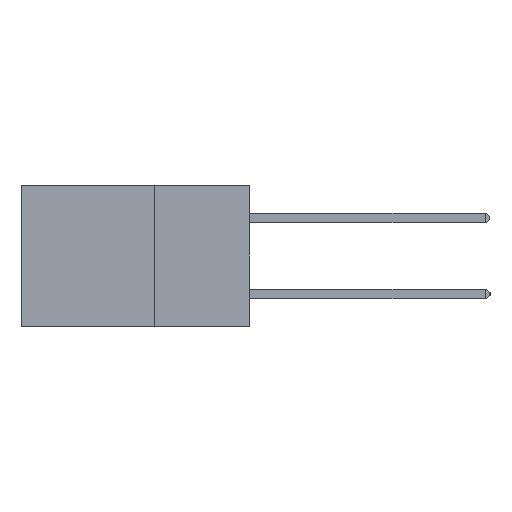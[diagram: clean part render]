
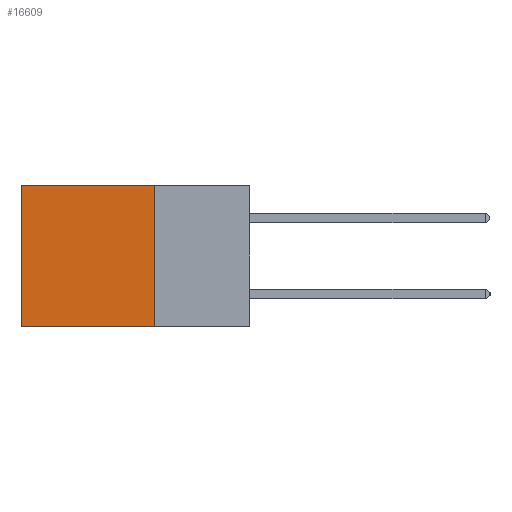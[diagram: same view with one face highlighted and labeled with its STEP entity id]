
A CAD part, left-side view. The second image highlights one B-rep face of the part: STEP entity #16609.
In plain terms, the highlighted planar face has unit normal (-1, 0, 0).
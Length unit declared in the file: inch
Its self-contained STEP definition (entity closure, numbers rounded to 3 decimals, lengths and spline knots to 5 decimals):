
#567 = VECTOR ( 'NONE', #21904, 39.37008 ) ;
#696 = ORIENTED_EDGE ( 'NONE', *, *, #16362, .F. ) ;
#1160 = ORIENTED_EDGE ( 'NONE', *, *, #2535, .T. ) ;
#2535 = EDGE_CURVE ( 'NONE', #18278, #21235, #11770, .T. ) ;
#5441 = FACE_OUTER_BOUND ( 'NONE', #7882, .T. ) ;
#5723 = VECTOR ( 'NONE', #8265, 39.37008 ) ;
#5736 = AXIS2_PLACEMENT_3D ( 'NONE', #21163, #8932, #21237 ) ;
#5966 = VECTOR ( 'NONE', #14530, 39.37008 ) ;
#7166 = PLANE ( 'NONE',  #5736 ) ;
#7882 = EDGE_LOOP ( 'NONE', ( #8597, #20189, #696, #1160 ) ) ;
#8265 = DIRECTION ( 'NONE',  ( 0., 0., -1. ) ) ;
#8451 = CARTESIAN_POINT ( 'NONE',  ( 0.2875, 0.6, 0. ) ) ;
#8597 = ORIENTED_EDGE ( 'NONE', *, *, #21418, .T. ) ;
#8932 = DIRECTION ( 'NONE',  ( 1., 0., 0. ) ) ;
#9014 = VECTOR ( 'NONE', #23054, 39.37008 ) ;
#10452 = LINE ( 'NONE', #17069, #5723 ) ;
#11082 = CARTESIAN_POINT ( 'NONE',  ( 0.2875, 0.25, 0. ) ) ;
#11751 = CARTESIAN_POINT ( 'NONE',  ( 0.2875, 0.25, -0.37 ) ) ;
#11770 = LINE ( 'NONE', #11082, #5966 ) ;
#14104 = VERTEX_POINT ( 'NONE', #11751 ) ;
#14530 = DIRECTION ( 'NONE',  ( 0., 1., 0. ) ) ;
#15516 = CARTESIAN_POINT ( 'NONE',  ( 0.2875, 0.25, 0. ) ) ;
#16312 = VERTEX_POINT ( 'NONE', #18747 ) ;
#16362 = EDGE_CURVE ( 'NONE', #18278, #14104, #10452, .T. ) ;
#16609 = ADVANCED_FACE ( 'NONE', ( #5441 ), #7166, .F. ) ;
#17069 = CARTESIAN_POINT ( 'NONE',  ( 0.2875, 0.25, 0. ) ) ;
#17927 = LINE ( 'NONE', #20151, #567 ) ;
#18278 = VERTEX_POINT ( 'NONE', #15516 ) ;
#18747 = CARTESIAN_POINT ( 'NONE',  ( 0.2875, 0.6, -0.37 ) ) ;
#18967 = LINE ( 'NONE', #21278, #9014 ) ;
#19136 = EDGE_CURVE ( 'NONE', #14104, #16312, #17927, .T. ) ;
#20151 = CARTESIAN_POINT ( 'NONE',  ( 0.2875, 0.25, -0.37 ) ) ;
#20189 = ORIENTED_EDGE ( 'NONE', *, *, #19136, .F. ) ;
#21163 = CARTESIAN_POINT ( 'NONE',  ( 0.2875, 0.25, 0. ) ) ;
#21235 = VERTEX_POINT ( 'NONE', #8451 ) ;
#21237 = DIRECTION ( 'NONE',  ( 0., 0., -1. ) ) ;
#21278 = CARTESIAN_POINT ( 'NONE',  ( 0.2875, 0.6, 0. ) ) ;
#21418 = EDGE_CURVE ( 'NONE', #21235, #16312, #18967, .T. ) ;
#21904 = DIRECTION ( 'NONE',  ( 0., 1., 0. ) ) ;
#23054 = DIRECTION ( 'NONE',  ( 0., 0., -1. ) ) ;
